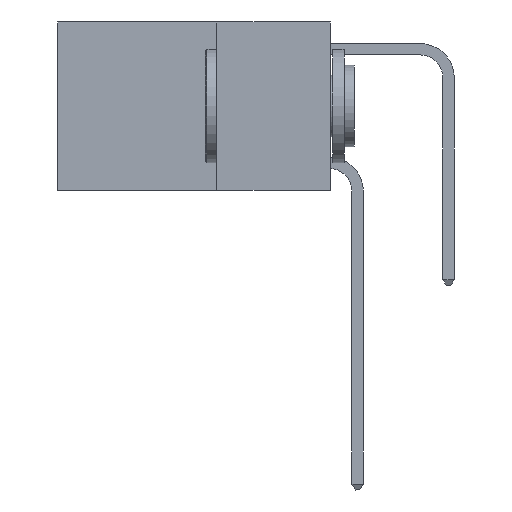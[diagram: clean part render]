
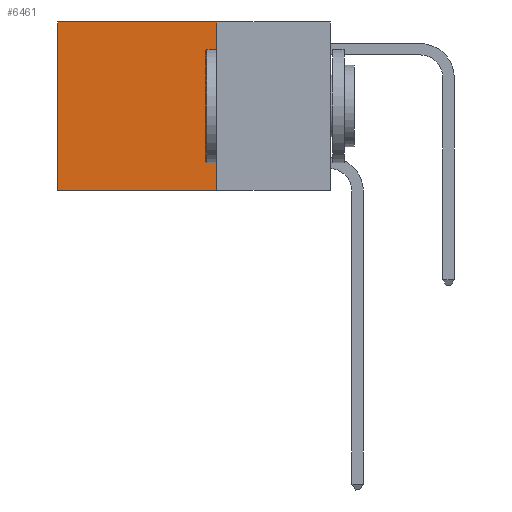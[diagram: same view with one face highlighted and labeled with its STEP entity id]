
A CAD part, left-side view. The second image highlights one B-rep face of the part: STEP entity #6461.
In plain terms, the highlighted planar face has unit normal (-1, 0, 0).
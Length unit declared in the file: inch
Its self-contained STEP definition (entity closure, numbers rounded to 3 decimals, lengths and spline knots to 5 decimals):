
#402 = LINE ( 'NONE', #7385, #7689 ) ;
#684 = DIRECTION ( 'NONE',  ( 0., 1., 0. ) ) ;
#951 = ORIENTED_EDGE ( 'NONE', *, *, #7420, .F. ) ;
#1074 = CARTESIAN_POINT ( 'NONE',  ( 0.2625, 0.25, 0. ) ) ;
#1444 = VERTEX_POINT ( 'NONE', #8532 ) ;
#1706 = ORIENTED_EDGE ( 'NONE', *, *, #4875, .F. ) ;
#2079 = CARTESIAN_POINT ( 'NONE',  ( 0.2625, 0.25, 0. ) ) ;
#2166 = LINE ( 'NONE', #2684, #4411 ) ;
#2499 = CARTESIAN_POINT ( 'NONE',  ( 0.2625, 0.25, -0.37 ) ) ;
#2684 = CARTESIAN_POINT ( 'NONE',  ( 0.2625, 0.25, 0. ) ) ;
#2793 = FACE_OUTER_BOUND ( 'NONE', #4681, .T. ) ;
#3034 = DIRECTION ( 'NONE',  ( 1., 0., 0. ) ) ;
#3360 = ORIENTED_EDGE ( 'NONE', *, *, #4946, .T. ) ;
#3590 = VERTEX_POINT ( 'NONE', #12065 ) ;
#3682 = DIRECTION ( 'NONE',  ( 0., 0., -1. ) ) ;
#4411 = VECTOR ( 'NONE', #5567, 39.37008 ) ;
#4681 = EDGE_LOOP ( 'NONE', ( #3360, #1706, #951, #11524 ) ) ;
#4875 = EDGE_CURVE ( 'NONE', #10054, #1444, #402, .T. ) ;
#4946 = EDGE_CURVE ( 'NONE', #8295, #1444, #9210, .T. ) ;
#5567 = DIRECTION ( 'NONE',  ( 0., 0., -1. ) ) ;
#5860 = VECTOR ( 'NONE', #8610, 39.37008 ) ;
#6461 = ADVANCED_FACE ( 'NONE', ( #2793 ), #7724, .F. ) ;
#6878 = VECTOR ( 'NONE', #3682, 39.37008 ) ;
#6887 = AXIS2_PLACEMENT_3D ( 'NONE', #2079, #3034, #9511 ) ;
#7385 = CARTESIAN_POINT ( 'NONE',  ( 0.2625, 0.25, -0.37 ) ) ;
#7420 = EDGE_CURVE ( 'NONE', #3590, #10054, #2166, .T. ) ;
#7689 = VECTOR ( 'NONE', #684, 39.37008 ) ;
#7724 = PLANE ( 'NONE',  #6887 ) ;
#8295 = VERTEX_POINT ( 'NONE', #8918 ) ;
#8532 = CARTESIAN_POINT ( 'NONE',  ( 0.2625, 0.6, -0.37 ) ) ;
#8610 = DIRECTION ( 'NONE',  ( 0., 1., 0. ) ) ;
#8918 = CARTESIAN_POINT ( 'NONE',  ( 0.2625, 0.6, 0. ) ) ;
#9182 = CARTESIAN_POINT ( 'NONE',  ( 0.2625, 0.6, 0. ) ) ;
#9210 = LINE ( 'NONE', #9182, #6878 ) ;
#9511 = DIRECTION ( 'NONE',  ( 0., 0., -1. ) ) ;
#9933 = LINE ( 'NONE', #1074, #5860 ) ;
#10054 = VERTEX_POINT ( 'NONE', #2499 ) ;
#10406 = EDGE_CURVE ( 'NONE', #3590, #8295, #9933, .T. ) ;
#11524 = ORIENTED_EDGE ( 'NONE', *, *, #10406, .T. ) ;
#12065 = CARTESIAN_POINT ( 'NONE',  ( 0.2625, 0.25, 0. ) ) ;
